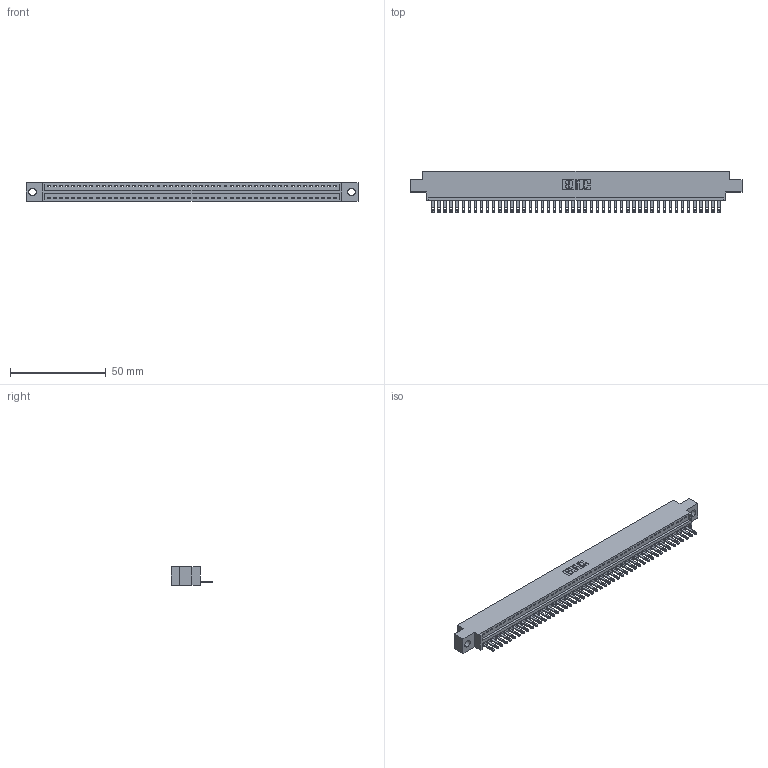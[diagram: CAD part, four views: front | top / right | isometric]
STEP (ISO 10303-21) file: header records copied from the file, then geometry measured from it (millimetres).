
FILE_DESCRIPTION (( 'STEP AP203' ), '1' );
FILE_NAME ('346-048-500-604.STEP', '2018-08-25T08:33:19', ( '' ), ( '' ), 'SwSTEP 2.0', 'SolidWorks 2016', '' );
FILE_SCHEMA (( 'CONFIG_CONTROL_DESIGN' ));
Length unit declared in the file: inch
Products named in the file (3): 346 Part_0.170 Offset - 0.156 Dia-TH; 345-292-001_345-293-100; 346-048-500-604
Assembly tree (49 placements, depth 2):
  346-048-500-604
    346 Part_0.170 Offset - 0.156 Dia-TH
    345-292-001_345-293-100  x48
Bounding box: 172.97 x 21.84 x 9.4 mm (x, y, z)
Volume: 16386 mm3; surface area: 20622.3 mm2
Topology: 49 solids, 49 shells, 2718 faces, 8405 edges, 5602 vertices
Faces by surface type: plane 1712, cylinder 1006
Entity records: 29047 total; most frequent: CARTESIAN_POINT 4984, ORIENTED_EDGE 4966, DIRECTION 4391, EDGE_CURVE 2483, LINE 2155, VECTOR 2155, VERTEX_POINT 1654, AXIS2_PLACEMENT_3D 1118
